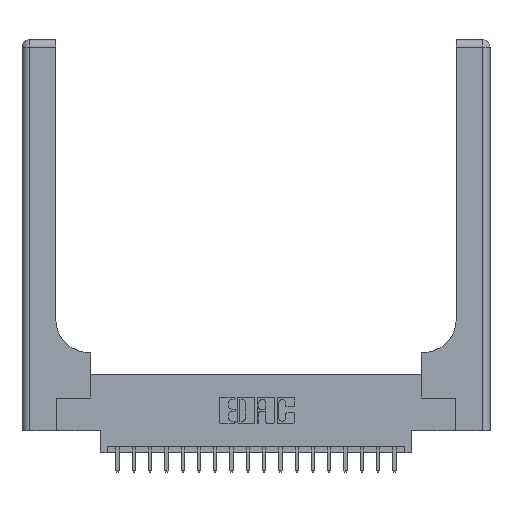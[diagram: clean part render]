
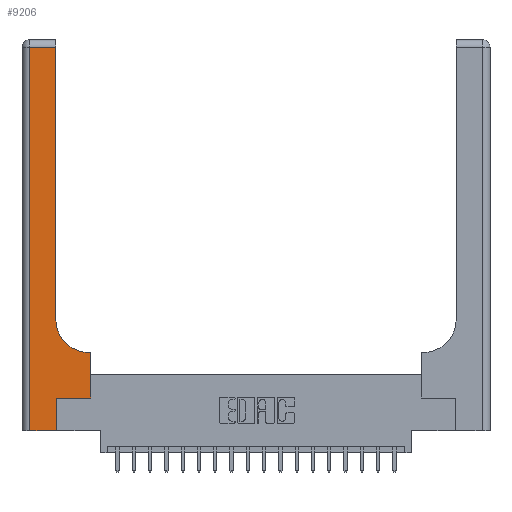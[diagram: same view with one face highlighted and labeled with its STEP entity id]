
A CAD part, top view. The second image highlights one B-rep face of the part: STEP entity #9206.
In plain terms, the highlighted planar face has unit normal (0, 0, 1).
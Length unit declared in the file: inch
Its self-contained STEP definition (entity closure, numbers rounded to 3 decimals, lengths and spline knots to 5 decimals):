
#1076 = CARTESIAN_POINT ( 'NONE',  ( 0.26, 2.94, 0.37 ) ) ;
#1411 = FACE_OUTER_BOUND ( 'NONE', #19984, .T. ) ;
#1467 = VERTEX_POINT ( 'NONE', #15765 ) ;
#1697 = ORIENTED_EDGE ( 'NONE', *, *, #14752, .T. ) ;
#1736 = ORIENTED_EDGE ( 'NONE', *, *, #17300, .T. ) ;
#1848 = VERTEX_POINT ( 'NONE', #18071 ) ;
#2185 = CARTESIAN_POINT ( 'NONE',  ( 0.26, 0.6, 0.37 ) ) ;
#2276 = EDGE_CURVE ( 'NONE', #17901, #8405, #6931, .T. ) ;
#2577 = AXIS2_PLACEMENT_3D ( 'NONE', #15694, #4473, #8884 ) ;
#2691 = CARTESIAN_POINT ( 'NONE',  ( 0.06, 2.94, 0.37 ) ) ;
#2942 = CARTESIAN_POINT ( 'NONE',  ( 0.06, 0., 0.37 ) ) ;
#3003 = DIRECTION ( 'NONE',  ( -1., 0., 0. ) ) ;
#3062 = DIRECTION ( 'NONE',  ( 0., -1., 0. ) ) ;
#3389 = EDGE_CURVE ( 'NONE', #7911, #11708, #4536, .T. ) ;
#3406 = CARTESIAN_POINT ( 'NONE',  ( 0.528, 0.25, 0.37 ) ) ;
#3546 = ORIENTED_EDGE ( 'NONE', *, *, #14911, .T. ) ;
#3745 = CARTESIAN_POINT ( 'NONE',  ( 0.265, 0.25, 0.37 ) ) ;
#3770 = CARTESIAN_POINT ( 'NONE',  ( 0.528, 0.6, 0.37 ) ) ;
#4063 = LINE ( 'NONE', #11966, #17086 ) ;
#4361 = CARTESIAN_POINT ( 'NONE',  ( 0.528, 0.25, 0.37 ) ) ;
#4473 = DIRECTION ( 'NONE',  ( 0., 0., -1. ) ) ;
#4536 = LINE ( 'NONE', #12433, #16949 ) ;
#4969 = ORIENTED_EDGE ( 'NONE', *, *, #10470, .T. ) ;
#5295 = AXIS2_PLACEMENT_3D ( 'NONE', #9290, #11191, #3003 ) ;
#5574 = CARTESIAN_POINT ( 'NONE',  ( 0., 0., 0.37 ) ) ;
#6559 = LINE ( 'NONE', #3406, #8962 ) ;
#6703 = DIRECTION ( 'NONE',  ( -1., 0., 0. ) ) ;
#6791 = EDGE_CURVE ( 'NONE', #1848, #1467, #19148, .T. ) ;
#6931 = LINE ( 'NONE', #2185, #14159 ) ;
#7514 = VECTOR ( 'NONE', #17166, 39.37008 ) ;
#7699 = EDGE_CURVE ( 'NONE', #1467, #12348, #13115, .T. ) ;
#7911 = VERTEX_POINT ( 'NONE', #2691 ) ;
#8405 = VERTEX_POINT ( 'NONE', #13368 ) ;
#8819 = ORIENTED_EDGE ( 'NONE', *, *, #6791, .T. ) ;
#8884 = DIRECTION ( 'NONE',  ( 1., 0., 0. ) ) ;
#8949 = CIRCLE ( 'NONE', #2577, 0.25 ) ;
#8962 = VECTOR ( 'NONE', #11083, 39.37008 ) ;
#9206 = ADVANCED_FACE ( 'NONE', ( #1411 ), #18941, .F. ) ;
#9290 = CARTESIAN_POINT ( 'NONE',  ( 0., 3., 0.37 ) ) ;
#9539 = VECTOR ( 'NONE', #6703, 39.37008 ) ;
#10470 = EDGE_CURVE ( 'NONE', #15198, #7911, #13017, .T. ) ;
#11083 = DIRECTION ( 'NONE',  ( 0., 1., 0. ) ) ;
#11191 = DIRECTION ( 'NONE',  ( 0., 0., -1. ) ) ;
#11257 = ORIENTED_EDGE ( 'NONE', *, *, #3389, .T. ) ;
#11689 = VECTOR ( 'NONE', #15223, 39.37008 ) ;
#11708 = VERTEX_POINT ( 'NONE', #2942 ) ;
#11785 = DIRECTION ( 'NONE',  ( -1., 0., 0. ) ) ;
#11966 = CARTESIAN_POINT ( 'NONE',  ( 0.26, 3., 0.37 ) ) ;
#12348 = VERTEX_POINT ( 'NONE', #4361 ) ;
#12433 = CARTESIAN_POINT ( 'NONE',  ( 0.06, 3., 0.37 ) ) ;
#13017 = LINE ( 'NONE', #13134, #9539 ) ;
#13115 = LINE ( 'NONE', #3745, #18117 ) ;
#13134 = CARTESIAN_POINT ( 'NONE',  ( 0., 2.94, 0.37 ) ) ;
#13368 = CARTESIAN_POINT ( 'NONE',  ( 0.51, 0.6, 0.37 ) ) ;
#14159 = VECTOR ( 'NONE', #11785, 39.37008 ) ;
#14752 = EDGE_CURVE ( 'NONE', #8405, #19241, #8949, .T. ) ;
#14911 = EDGE_CURVE ( 'NONE', #12348, #17901, #6559, .T. ) ;
#15198 = VERTEX_POINT ( 'NONE', #1076 ) ;
#15223 = DIRECTION ( 'NONE',  ( 1., 0., 0. ) ) ;
#15694 = CARTESIAN_POINT ( 'NONE',  ( 0.51, 0.85, 0.37 ) ) ;
#15765 = CARTESIAN_POINT ( 'NONE',  ( 0.265, 0.25, 0.37 ) ) ;
#15899 = CARTESIAN_POINT ( 'NONE',  ( 0.265, 0., 0.37 ) ) ;
#15948 = ORIENTED_EDGE ( 'NONE', *, *, #2276, .T. ) ;
#16334 = ORIENTED_EDGE ( 'NONE', *, *, #19728, .T. ) ;
#16583 = CARTESIAN_POINT ( 'NONE',  ( 0.26, 0.85, 0.37 ) ) ;
#16793 = LINE ( 'NONE', #5574, #11689 ) ;
#16949 = VECTOR ( 'NONE', #3062, 39.37008 ) ;
#17086 = VECTOR ( 'NONE', #19909, 39.37008 ) ;
#17166 = DIRECTION ( 'NONE',  ( 0., 1., 0. ) ) ;
#17300 = EDGE_CURVE ( 'NONE', #11708, #1848, #16793, .T. ) ;
#17901 = VERTEX_POINT ( 'NONE', #3770 ) ;
#18071 = CARTESIAN_POINT ( 'NONE',  ( 0.265, 0., 0.37 ) ) ;
#18117 = VECTOR ( 'NONE', #19903, 39.37008 ) ;
#18306 = ORIENTED_EDGE ( 'NONE', *, *, #7699, .T. ) ;
#18941 = PLANE ( 'NONE',  #5295 ) ;
#19148 = LINE ( 'NONE', #15899, #7514 ) ;
#19241 = VERTEX_POINT ( 'NONE', #16583 ) ;
#19728 = EDGE_CURVE ( 'NONE', #19241, #15198, #4063, .T. ) ;
#19903 = DIRECTION ( 'NONE',  ( 1., 0., 0. ) ) ;
#19909 = DIRECTION ( 'NONE',  ( 0., 1., 0. ) ) ;
#19984 = EDGE_LOOP ( 'NONE', ( #16334, #4969, #11257, #1736, #8819, #18306, #3546, #15948, #1697 ) ) ;
